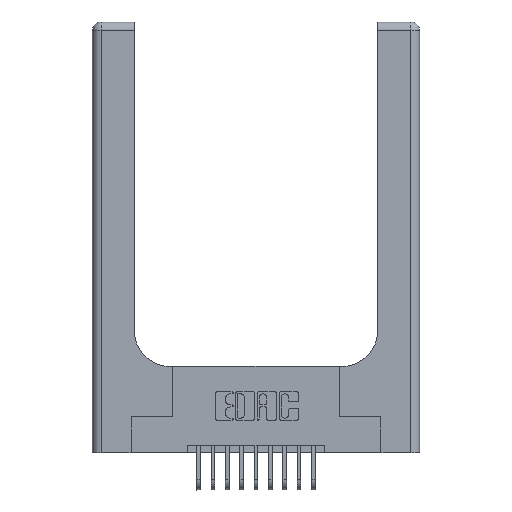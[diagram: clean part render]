
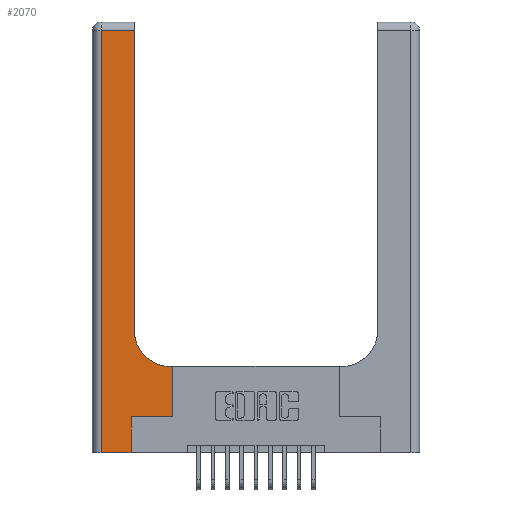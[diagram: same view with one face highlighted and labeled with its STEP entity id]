
A CAD part, top view. The second image highlights one B-rep face of the part: STEP entity #2070.
In plain terms, the highlighted planar face has unit normal (0, 0, 1).
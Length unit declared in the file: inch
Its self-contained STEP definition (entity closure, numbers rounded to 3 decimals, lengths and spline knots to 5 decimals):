
#198 = VERTEX_POINT ( 'NONE', #3709 ) ;
#234 = PLANE ( 'NONE',  #14178 ) ;
#280 = VERTEX_POINT ( 'NONE', #16427 ) ;
#297 = LINE ( 'NONE', #13406, #3349 ) ;
#384 = CARTESIAN_POINT ( 'NONE',  ( 0.06, 0., 0.37 ) ) ;
#414 = DIRECTION ( 'NONE',  ( -1., 0., 0. ) ) ;
#682 = CARTESIAN_POINT ( 'NONE',  ( 0.2915, 0.6, 0.37 ) ) ;
#879 = EDGE_CURVE ( 'NONE', #3719, #280, #16023, .T. ) ;
#1459 = VECTOR ( 'NONE', #7737, 39.37008 ) ;
#1572 = DIRECTION ( 'NONE',  ( 0., 0., -1. ) ) ;
#1578 = LINE ( 'NONE', #5681, #7928 ) ;
#1712 = ORIENTED_EDGE ( 'NONE', *, *, #4552, .T. ) ;
#1726 = EDGE_CURVE ( 'NONE', #280, #14575, #9047, .T. ) ;
#1785 = CARTESIAN_POINT ( 'NONE',  ( 0.269, 0.25, 0.37 ) ) ;
#1894 = VERTEX_POINT ( 'NONE', #13890 ) ;
#2070 = ADVANCED_FACE ( 'NONE', ( #13840 ), #234, .F. ) ;
#2268 = CARTESIAN_POINT ( 'NONE',  ( 0.2915, 0.85, 0.37 ) ) ;
#2290 = DIRECTION ( 'NONE',  ( 1., 0., 0. ) ) ;
#2335 = ORIENTED_EDGE ( 'NONE', *, *, #1726, .T. ) ;
#2337 = CARTESIAN_POINT ( 'NONE',  ( 0.06, 3., 0.37 ) ) ;
#2843 = LINE ( 'NONE', #2337, #15906 ) ;
#2876 = LINE ( 'NONE', #9839, #12948 ) ;
#3255 = ORIENTED_EDGE ( 'NONE', *, *, #12947, .T. ) ;
#3349 = VECTOR ( 'NONE', #12118, 39.37008 ) ;
#3487 = CARTESIAN_POINT ( 'NONE',  ( 0.5415, 0.85, 0.37 ) ) ;
#3648 = CARTESIAN_POINT ( 'NONE',  ( 0.5585, 0.6, 0.37 ) ) ;
#3709 = CARTESIAN_POINT ( 'NONE',  ( 0.269, 0., 0.37 ) ) ;
#3719 = VERTEX_POINT ( 'NONE', #3648 ) ;
#4552 = EDGE_CURVE ( 'NONE', #13793, #14082, #2876, .T. ) ;
#4726 = DIRECTION ( 'NONE',  ( 1., 0., 0. ) ) ;
#5025 = ORIENTED_EDGE ( 'NONE', *, *, #10112, .T. ) ;
#5342 = DIRECTION ( 'NONE',  ( 0., 1., 0. ) ) ;
#5494 = ORIENTED_EDGE ( 'NONE', *, *, #14047, .T. ) ;
#5557 = VECTOR ( 'NONE', #15849, 39.37008 ) ;
#5681 = CARTESIAN_POINT ( 'NONE',  ( 0., 0., 0.37 ) ) ;
#6255 = CARTESIAN_POINT ( 'NONE',  ( 0.5585, 0.25, 0.37 ) ) ;
#6983 = DIRECTION ( 'NONE',  ( 1., 0., 0. ) ) ;
#7511 = CARTESIAN_POINT ( 'NONE',  ( 0.06, 2.94, 0.37 ) ) ;
#7737 = DIRECTION ( 'NONE',  ( 0., 1., 0. ) ) ;
#7896 = CARTESIAN_POINT ( 'NONE',  ( 0., 3., 0.37 ) ) ;
#7928 = VECTOR ( 'NONE', #6983, 39.37008 ) ;
#8141 = ORIENTED_EDGE ( 'NONE', *, *, #10677, .T. ) ;
#8189 = LINE ( 'NONE', #15341, #1459 ) ;
#8301 = VERTEX_POINT ( 'NONE', #384 ) ;
#8437 = EDGE_LOOP ( 'NONE', ( #5025, #8141, #5494, #14491, #11421, #1712, #3255, #16066, #2335 ) ) ;
#8706 = VERTEX_POINT ( 'NONE', #7511 ) ;
#9047 = CIRCLE ( 'NONE', #9368, 0.25 ) ;
#9115 = CARTESIAN_POINT ( 'NONE',  ( 0.2915, 3., 0.37 ) ) ;
#9368 = AXIS2_PLACEMENT_3D ( 'NONE', #3487, #12306, #4726 ) ;
#9707 = EDGE_CURVE ( 'NONE', #8301, #198, #1578, .T. ) ;
#9839 = CARTESIAN_POINT ( 'NONE',  ( 0.269, 0.25, 0.37 ) ) ;
#10112 = EDGE_CURVE ( 'NONE', #14575, #1894, #15052, .T. ) ;
#10402 = DIRECTION ( 'NONE',  ( -1., 0., 0. ) ) ;
#10677 = EDGE_CURVE ( 'NONE', #1894, #8706, #297, .T. ) ;
#11421 = ORIENTED_EDGE ( 'NONE', *, *, #14360, .T. ) ;
#12118 = DIRECTION ( 'NONE',  ( -1., 0., 0. ) ) ;
#12306 = DIRECTION ( 'NONE',  ( 0., 0., -1. ) ) ;
#12638 = VECTOR ( 'NONE', #414, 39.37008 ) ;
#12947 = EDGE_CURVE ( 'NONE', #14082, #3719, #8189, .T. ) ;
#12948 = VECTOR ( 'NONE', #2290, 39.37008 ) ;
#13406 = CARTESIAN_POINT ( 'NONE',  ( 0., 2.94, 0.37 ) ) ;
#13793 = VERTEX_POINT ( 'NONE', #1785 ) ;
#13840 = FACE_OUTER_BOUND ( 'NONE', #8437, .T. ) ;
#13890 = CARTESIAN_POINT ( 'NONE',  ( 0.2915, 2.94, 0.37 ) ) ;
#14047 = EDGE_CURVE ( 'NONE', #8706, #8301, #2843, .T. ) ;
#14082 = VERTEX_POINT ( 'NONE', #6255 ) ;
#14178 = AXIS2_PLACEMENT_3D ( 'NONE', #7896, #1572, #10402 ) ;
#14360 = EDGE_CURVE ( 'NONE', #198, #13793, #15707, .T. ) ;
#14491 = ORIENTED_EDGE ( 'NONE', *, *, #9707, .T. ) ;
#14575 = VERTEX_POINT ( 'NONE', #2268 ) ;
#14585 = CARTESIAN_POINT ( 'NONE',  ( 0.269, 0., 0.37 ) ) ;
#14665 = VECTOR ( 'NONE', #5342, 39.37008 ) ;
#15052 = LINE ( 'NONE', #9115, #14665 ) ;
#15341 = CARTESIAN_POINT ( 'NONE',  ( 0.5585, 0.25, 0.37 ) ) ;
#15707 = LINE ( 'NONE', #14585, #5557 ) ;
#15849 = DIRECTION ( 'NONE',  ( 0., 1., 0. ) ) ;
#15906 = VECTOR ( 'NONE', #16292, 39.37008 ) ;
#16023 = LINE ( 'NONE', #682, #12638 ) ;
#16066 = ORIENTED_EDGE ( 'NONE', *, *, #879, .T. ) ;
#16292 = DIRECTION ( 'NONE',  ( 0., -1., 0. ) ) ;
#16427 = CARTESIAN_POINT ( 'NONE',  ( 0.5415, 0.6, 0.37 ) ) ;
